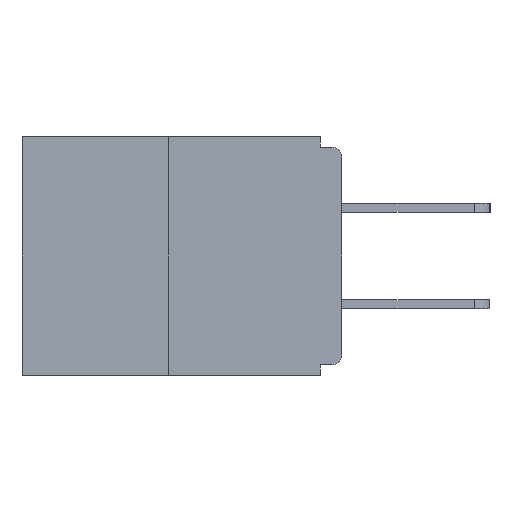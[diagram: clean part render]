
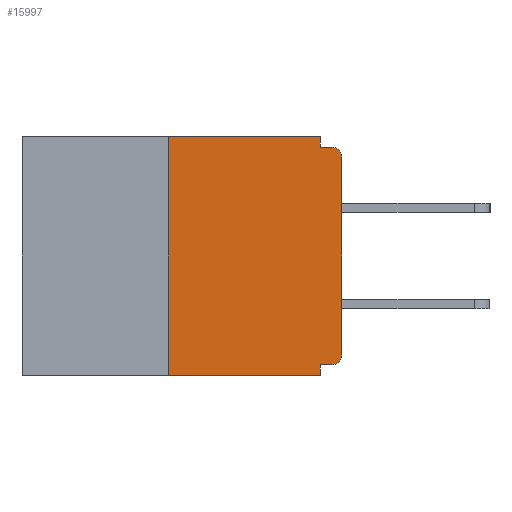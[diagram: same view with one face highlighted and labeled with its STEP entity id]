
A CAD part, left-side view. The second image highlights one B-rep face of the part: STEP entity #15997.
In plain terms, the highlighted planar face has unit normal (-1, 0, 0).
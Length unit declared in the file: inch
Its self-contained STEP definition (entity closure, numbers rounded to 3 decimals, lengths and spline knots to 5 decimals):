
#911 = ORIENTED_EDGE ( 'NONE', *, *, #17297, .F. ) ;
#947 = AXIS2_PLACEMENT_3D ( 'NONE', #27755, #7374, #16463 ) ;
#977 = PLANE ( 'NONE',  #21403 ) ;
#1223 = CARTESIAN_POINT ( 'NONE',  ( 0., 0.015, -0.015 ) ) ;
#1314 = CARTESIAN_POINT ( 'NONE',  ( 0., 0., 0. ) ) ;
#1599 = VECTOR ( 'NONE', #14830, 39.37008 ) ;
#2074 = CARTESIAN_POINT ( 'NONE',  ( 0., 0.015, -0.328 ) ) ;
#2491 = CARTESIAN_POINT ( 'NONE',  ( 0., 0.031, -0.343 ) ) ;
#2939 = EDGE_CURVE ( 'NONE', #5350, #26346, #3398, .T. ) ;
#3398 = LINE ( 'NONE', #14727, #11776 ) ;
#3818 = ORIENTED_EDGE ( 'NONE', *, *, #22623, .F. ) ;
#3829 = LINE ( 'NONE', #10844, #13324 ) ;
#3876 = EDGE_CURVE ( 'NONE', #24701, #7392, #3829, .T. ) ;
#4942 = FACE_OUTER_BOUND ( 'NONE', #11569, .T. ) ;
#5025 = LINE ( 'NONE', #17981, #15664 ) ;
#5173 = ORIENTED_EDGE ( 'NONE', *, *, #18542, .T. ) ;
#5350 = VERTEX_POINT ( 'NONE', #24975 ) ;
#5725 = LINE ( 'NONE', #13010, #26515 ) ;
#5750 = LINE ( 'NONE', #28515, #1599 ) ;
#6336 = EDGE_CURVE ( 'NONE', #10526, #25937, #6928, .T. ) ;
#6820 = ORIENTED_EDGE ( 'NONE', *, *, #6336, .T. ) ;
#6928 = LINE ( 'NONE', #25393, #7304 ) ;
#6982 = LINE ( 'NONE', #2491, #21105 ) ;
#7304 = VECTOR ( 'NONE', #25083, 39.37008 ) ;
#7374 = DIRECTION ( 'NONE',  ( -1., 0., 0. ) ) ;
#7392 = VERTEX_POINT ( 'NONE', #19325 ) ;
#7403 = EDGE_CURVE ( 'NONE', #10526, #24701, #5750, .T. ) ;
#10526 = VERTEX_POINT ( 'NONE', #18824 ) ;
#10704 = VERTEX_POINT ( 'NONE', #12968 ) ;
#10844 = CARTESIAN_POINT ( 'NONE',  ( 0., 0.46, 0. ) ) ;
#10993 = DIRECTION ( 'NONE',  ( 0., 0., -1. ) ) ;
#11569 = EDGE_LOOP ( 'NONE', ( #24905, #12864, #6820, #3818, #12207, #5173, #22501, #12550, #21058, #911 ) ) ;
#11776 = VECTOR ( 'NONE', #14574, 39.37008 ) ;
#12207 = ORIENTED_EDGE ( 'NONE', *, *, #27687, .F. ) ;
#12550 = ORIENTED_EDGE ( 'NONE', *, *, #20182, .T. ) ;
#12864 = ORIENTED_EDGE ( 'NONE', *, *, #7403, .F. ) ;
#12968 = CARTESIAN_POINT ( 'NONE',  ( 0., 0.031, -0.328 ) ) ;
#13010 = CARTESIAN_POINT ( 'NONE',  ( 0., 0., -0.328 ) ) ;
#13324 = VECTOR ( 'NONE', #26470, 39.37008 ) ;
#14371 = VERTEX_POINT ( 'NONE', #17572 ) ;
#14574 = DIRECTION ( 'NONE',  ( 0., -1., 0. ) ) ;
#14727 = CARTESIAN_POINT ( 'NONE',  ( 0., 0., -0.015 ) ) ;
#14749 = DIRECTION ( 'NONE',  ( 0., 0., 1. ) ) ;
#14830 = DIRECTION ( 'NONE',  ( 0., 0., 1. ) ) ;
#15664 = VECTOR ( 'NONE', #27029, 39.37008 ) ;
#15997 = ADVANCED_FACE ( 'NONE', ( #4942 ), #977, .F. ) ;
#16274 = CARTESIAN_POINT ( 'NONE',  ( 0., 0.015, -0.03 ) ) ;
#16463 = DIRECTION ( 'NONE',  ( 0., 0., -1. ) ) ;
#17297 = EDGE_CURVE ( 'NONE', #7392, #5350, #5025, .T. ) ;
#17425 = VECTOR ( 'NONE', #14749, 39.37008 ) ;
#17572 = CARTESIAN_POINT ( 'NONE',  ( 0., 0., -0.313 ) ) ;
#17981 = CARTESIAN_POINT ( 'NONE',  ( 0., 0.031, 0. ) ) ;
#18542 = EDGE_CURVE ( 'NONE', #26810, #14371, #26651, .T. ) ;
#18824 = CARTESIAN_POINT ( 'NONE',  ( 0., 0.25, -0.343 ) ) ;
#19202 = CARTESIAN_POINT ( 'NONE',  ( 0., 0.46, 0. ) ) ;
#19325 = CARTESIAN_POINT ( 'NONE',  ( 0., 0.031, 0. ) ) ;
#19341 = DIRECTION ( 'NONE',  ( 1., 0., 0. ) ) ;
#20182 = EDGE_CURVE ( 'NONE', #29324, #26346, #27688, .T. ) ;
#21058 = ORIENTED_EDGE ( 'NONE', *, *, #2939, .F. ) ;
#21105 = VECTOR ( 'NONE', #10993, 39.37008 ) ;
#21188 = DIRECTION ( 'NONE',  ( -1., 0., 0. ) ) ;
#21403 = AXIS2_PLACEMENT_3D ( 'NONE', #19202, #19341, #25036 ) ;
#21519 = AXIS2_PLACEMENT_3D ( 'NONE', #16274, #21188, #27424 ) ;
#21748 = LINE ( 'NONE', #1314, #17425 ) ;
#22501 = ORIENTED_EDGE ( 'NONE', *, *, #25468, .T. ) ;
#22623 = EDGE_CURVE ( 'NONE', #10704, #25937, #6982, .T. ) ;
#23955 = CARTESIAN_POINT ( 'NONE',  ( 0., 0.031, -0.343 ) ) ;
#24346 = CARTESIAN_POINT ( 'NONE',  ( 0., 0.25, 0. ) ) ;
#24701 = VERTEX_POINT ( 'NONE', #24346 ) ;
#24905 = ORIENTED_EDGE ( 'NONE', *, *, #3876, .F. ) ;
#24975 = CARTESIAN_POINT ( 'NONE',  ( 0., 0.031, -0.015 ) ) ;
#25036 = DIRECTION ( 'NONE',  ( 0., 0., -1. ) ) ;
#25083 = DIRECTION ( 'NONE',  ( 0., -1., 0. ) ) ;
#25393 = CARTESIAN_POINT ( 'NONE',  ( 0., 0.46, -0.343 ) ) ;
#25468 = EDGE_CURVE ( 'NONE', #14371, #29324, #21748, .T. ) ;
#25937 = VERTEX_POINT ( 'NONE', #23955 ) ;
#26346 = VERTEX_POINT ( 'NONE', #1223 ) ;
#26470 = DIRECTION ( 'NONE',  ( 0., -1., 0. ) ) ;
#26515 = VECTOR ( 'NONE', #28491, 39.37008 ) ;
#26651 = CIRCLE ( 'NONE', #947, 0.015 ) ;
#26810 = VERTEX_POINT ( 'NONE', #2074 ) ;
#27029 = DIRECTION ( 'NONE',  ( 0., 0., -1. ) ) ;
#27424 = DIRECTION ( 'NONE',  ( 0., 0., -1. ) ) ;
#27687 = EDGE_CURVE ( 'NONE', #26810, #10704, #5725, .T. ) ;
#27688 = CIRCLE ( 'NONE', #21519, 0.015 ) ;
#27755 = CARTESIAN_POINT ( 'NONE',  ( 0., 0.015, -0.313 ) ) ;
#27945 = CARTESIAN_POINT ( 'NONE',  ( 0., 0., -0.03 ) ) ;
#28491 = DIRECTION ( 'NONE',  ( 0., 1., 0. ) ) ;
#28515 = CARTESIAN_POINT ( 'NONE',  ( 0., 0.25, 0. ) ) ;
#29324 = VERTEX_POINT ( 'NONE', #27945 ) ;
